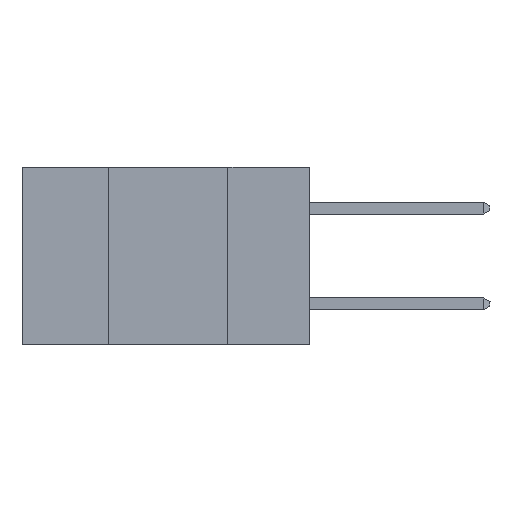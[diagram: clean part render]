
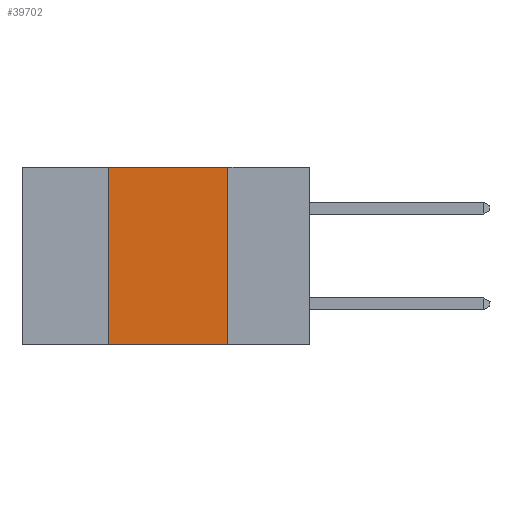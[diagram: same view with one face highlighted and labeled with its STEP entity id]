
A CAD part, left-side view. The second image highlights one B-rep face of the part: STEP entity #39702.
In plain terms, the highlighted planar face has unit normal (-1, 0, 0).
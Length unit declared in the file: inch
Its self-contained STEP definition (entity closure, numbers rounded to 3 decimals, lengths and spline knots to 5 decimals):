
#644 = ORIENTED_EDGE ( 'NONE', *, *, #17986, .F. ) ;
#3306 = CARTESIAN_POINT ( 'NONE',  ( 0., 0.6, -0.37 ) ) ;
#3775 = VECTOR ( 'NONE', #21792, 39.37008 ) ;
#4109 = DIRECTION ( 'NONE',  ( 0., 0., -1. ) ) ;
#6206 = DIRECTION ( 'NONE',  ( 0., -1., 0. ) ) ;
#7518 = VERTEX_POINT ( 'NONE', #42444 ) ;
#8240 = CARTESIAN_POINT ( 'NONE',  ( 0., 0.42, 0. ) ) ;
#10912 = AXIS2_PLACEMENT_3D ( 'NONE', #12997, #33903, #27217 ) ;
#12841 = VERTEX_POINT ( 'NONE', #8240 ) ;
#12997 = CARTESIAN_POINT ( 'NONE',  ( 0., 0.6, 0. ) ) ;
#14881 = EDGE_LOOP ( 'NONE', ( #19368, #28083, #644, #28099 ) ) ;
#15005 = VERTEX_POINT ( 'NONE', #34212 ) ;
#17473 = CARTESIAN_POINT ( 'NONE',  ( 0., 0.17, 0. ) ) ;
#17986 = EDGE_CURVE ( 'NONE', #15005, #12841, #28891, .T. ) ;
#19159 = CARTESIAN_POINT ( 'NONE',  ( 0., 0.17, 0. ) ) ;
#19368 = ORIENTED_EDGE ( 'NONE', *, *, #20999, .F. ) ;
#20116 = FACE_OUTER_BOUND ( 'NONE', #14881, .T. ) ;
#20198 = EDGE_CURVE ( 'NONE', #12841, #37194, #37610, .T. ) ;
#20999 = EDGE_CURVE ( 'NONE', #37194, #7518, #37781, .T. ) ;
#21792 = DIRECTION ( 'NONE',  ( 0., 0., 1. ) ) ;
#23459 = PLANE ( 'NONE',  #10912 ) ;
#27217 = DIRECTION ( 'NONE',  ( 0., 0., -1. ) ) ;
#27434 = EDGE_CURVE ( 'NONE', #15005, #7518, #40040, .T. ) ;
#27959 = VECTOR ( 'NONE', #30721, 39.37008 ) ;
#28083 = ORIENTED_EDGE ( 'NONE', *, *, #20198, .F. ) ;
#28099 = ORIENTED_EDGE ( 'NONE', *, *, #27434, .T. ) ;
#28891 = LINE ( 'NONE', #42459, #3775 ) ;
#30689 = VECTOR ( 'NONE', #6206, 39.37008 ) ;
#30721 = DIRECTION ( 'NONE',  ( 0., -1., 0. ) ) ;
#32273 = VECTOR ( 'NONE', #4109, 39.37008 ) ;
#33903 = DIRECTION ( 'NONE',  ( 1., 0., 0. ) ) ;
#34212 = CARTESIAN_POINT ( 'NONE',  ( 0., 0.42, -0.37 ) ) ;
#37194 = VERTEX_POINT ( 'NONE', #19159 ) ;
#37610 = LINE ( 'NONE', #38050, #27959 ) ;
#37781 = LINE ( 'NONE', #17473, #32273 ) ;
#38050 = CARTESIAN_POINT ( 'NONE',  ( 0., 0.6, 0. ) ) ;
#39702 = ADVANCED_FACE ( 'NONE', ( #20116 ), #23459, .F. ) ;
#40040 = LINE ( 'NONE', #3306, #30689 ) ;
#42444 = CARTESIAN_POINT ( 'NONE',  ( 0., 0.17, -0.37 ) ) ;
#42459 = CARTESIAN_POINT ( 'NONE',  ( 0., 0.42, 0. ) ) ;
